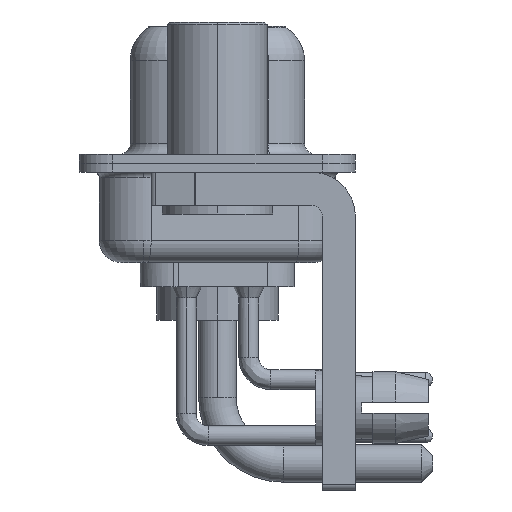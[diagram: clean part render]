
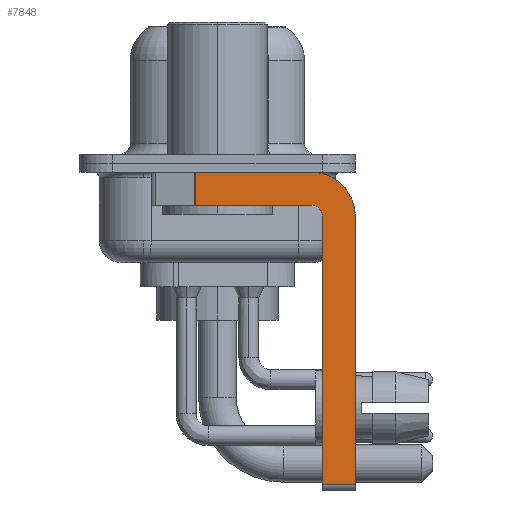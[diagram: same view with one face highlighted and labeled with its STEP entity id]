
A CAD part, left-side view. The second image highlights one B-rep face of the part: STEP entity #7848.
In plain terms, the highlighted planar face has unit normal (-1, 0, 0).
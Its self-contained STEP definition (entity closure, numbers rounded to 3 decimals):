
#491 = CARTESIAN_POINT ( 'NONE',  ( -2.9, -4.25, -2.4 ) ) ;
#566 = DIRECTION ( 'NONE',  ( 0., 0., 1. ) ) ;
#687 = CARTESIAN_POINT ( 'NONE',  ( -2.9, -4.25, -1.9 ) ) ;
#1500 = VERTEX_POINT ( 'NONE', #18346 ) ;
#2022 = EDGE_LOOP ( 'NONE', ( #25664, #7149, #22198, #9344, #16320, #15491, #9780, #16236 ) ) ;
#2594 = DIRECTION ( 'NONE',  ( 1., 0., 0. ) ) ;
#3237 = DIRECTION ( 'NONE',  ( -1., 0., 0. ) ) ;
#3957 = CARTESIAN_POINT ( 'NONE',  ( -2.9, -4.25, -1.9 ) ) ;
#4274 = LINE ( 'NONE', #20447, #21246 ) ;
#5084 = CARTESIAN_POINT ( 'NONE',  ( -2.9, -4.25, -14.55 ) ) ;
#5457 = EDGE_CURVE ( 'NONE', #6266, #16176, #7677, .T. ) ;
#6266 = VERTEX_POINT ( 'NONE', #15510 ) ;
#6464 = DIRECTION ( 'NONE',  ( 0., 0., -1. ) ) ;
#6520 = VERTEX_POINT ( 'NONE', #22484 ) ;
#7149 = ORIENTED_EDGE ( 'NONE', *, *, #5457, .T. ) ;
#7677 = LINE ( 'NONE', #7946, #8189 ) ;
#7848 = ADVANCED_FACE ( 'NONE', ( #22879 ), #16547, .F. ) ;
#7946 = CARTESIAN_POINT ( 'NONE',  ( -2.9, 0.978, -1.9 ) ) ;
#8126 = CIRCLE ( 'NONE', #22935, 0.5 ) ;
#8189 = VECTOR ( 'NONE', #15775, 1000. ) ;
#8742 = VECTOR ( 'NONE', #15000, 1000. ) ;
#9344 = ORIENTED_EDGE ( 'NONE', *, *, #11036, .F. ) ;
#9355 = AXIS2_PLACEMENT_3D ( 'NONE', #20886, #2594, #24715 ) ;
#9605 = VERTEX_POINT ( 'NONE', #16142 ) ;
#9780 = ORIENTED_EDGE ( 'NONE', *, *, #19954, .F. ) ;
#10449 = DIRECTION ( 'NONE',  ( 1., 0., 0. ) ) ;
#11036 = EDGE_CURVE ( 'NONE', #6520, #12692, #8126, .T. ) ;
#11779 = LINE ( 'NONE', #23426, #14109 ) ;
#12692 = VERTEX_POINT ( 'NONE', #3957 ) ;
#13031 = DIRECTION ( 'NONE',  ( 0., -1., 0. ) ) ;
#13902 = EDGE_CURVE ( 'NONE', #6266, #1500, #24934, .T. ) ;
#14109 = VECTOR ( 'NONE', #19737, 1000. ) ;
#15000 = DIRECTION ( 'NONE',  ( 0., 1., 0. ) ) ;
#15086 = CARTESIAN_POINT ( 'NONE',  ( -2.9, 0.978, -1.9 ) ) ;
#15148 = EDGE_CURVE ( 'NONE', #12692, #16176, #19231, .T. ) ;
#15187 = VERTEX_POINT ( 'NONE', #17250 ) ;
#15465 = AXIS2_PLACEMENT_3D ( 'NONE', #491, #10449, #6464 ) ;
#15491 = ORIENTED_EDGE ( 'NONE', *, *, #19413, .T. ) ;
#15510 = CARTESIAN_POINT ( 'NONE',  ( -2.9, 0.978, -0.4 ) ) ;
#15563 = LINE ( 'NONE', #5084, #18295 ) ;
#15775 = DIRECTION ( 'NONE',  ( 0., 0., -1. ) ) ;
#16142 = CARTESIAN_POINT ( 'NONE',  ( -2.9, -4.75, -14.55 ) ) ;
#16176 = VERTEX_POINT ( 'NONE', #15086 ) ;
#16236 = ORIENTED_EDGE ( 'NONE', *, *, #18130, .F. ) ;
#16320 = ORIENTED_EDGE ( 'NONE', *, *, #17291, .F. ) ;
#16547 = PLANE ( 'NONE',  #15465 ) ;
#16568 = CIRCLE ( 'NONE', #9355, 2. ) ;
#17250 = CARTESIAN_POINT ( 'NONE',  ( -2.9, -6.25, -2.4 ) ) ;
#17291 = EDGE_CURVE ( 'NONE', #9605, #6520, #4274, .T. ) ;
#18130 = EDGE_CURVE ( 'NONE', #1500, #15187, #16568, .T. ) ;
#18295 = VECTOR ( 'NONE', #25235, 1000. ) ;
#18346 = CARTESIAN_POINT ( 'NONE',  ( -2.9, -4.25, -0.4 ) ) ;
#18424 = VECTOR ( 'NONE', #13031, 1000. ) ;
#19231 = LINE ( 'NONE', #687, #8742 ) ;
#19413 = EDGE_CURVE ( 'NONE', #9605, #25117, #15563, .T. ) ;
#19737 = DIRECTION ( 'NONE',  ( 0., 0., -1. ) ) ;
#19793 = CARTESIAN_POINT ( 'NONE',  ( -2.9, -4.25, -2.4 ) ) ;
#19954 = EDGE_CURVE ( 'NONE', #15187, #25117, #11779, .T. ) ;
#20140 = CARTESIAN_POINT ( 'NONE',  ( -2.9, -6.25, -14.55 ) ) ;
#20447 = CARTESIAN_POINT ( 'NONE',  ( -2.9, -4.75, -14.8 ) ) ;
#20886 = CARTESIAN_POINT ( 'NONE',  ( -2.9, -4.25, -2.4 ) ) ;
#21246 = VECTOR ( 'NONE', #566, 1000. ) ;
#22198 = ORIENTED_EDGE ( 'NONE', *, *, #15148, .F. ) ;
#22484 = CARTESIAN_POINT ( 'NONE',  ( -2.9, -4.75, -2.4 ) ) ;
#22879 = FACE_OUTER_BOUND ( 'NONE', #2022, .T. ) ;
#22935 = AXIS2_PLACEMENT_3D ( 'NONE', #19793, #3237, #23621 ) ;
#22944 = CARTESIAN_POINT ( 'NONE',  ( -2.9, 3., -0.4 ) ) ;
#23426 = CARTESIAN_POINT ( 'NONE',  ( -2.9, -6.25, -2.4 ) ) ;
#23621 = DIRECTION ( 'NONE',  ( 0., 0., 1. ) ) ;
#24715 = DIRECTION ( 'NONE',  ( 0., 0., -1. ) ) ;
#24934 = LINE ( 'NONE', #22944, #18424 ) ;
#25117 = VERTEX_POINT ( 'NONE', #20140 ) ;
#25235 = DIRECTION ( 'NONE',  ( 0., -1., 0. ) ) ;
#25664 = ORIENTED_EDGE ( 'NONE', *, *, #13902, .F. ) ;
